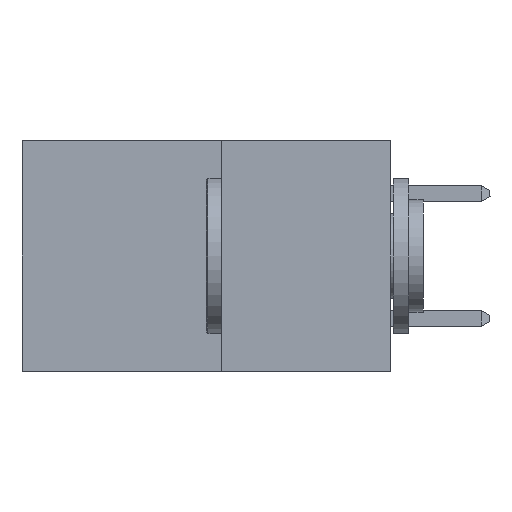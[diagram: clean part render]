
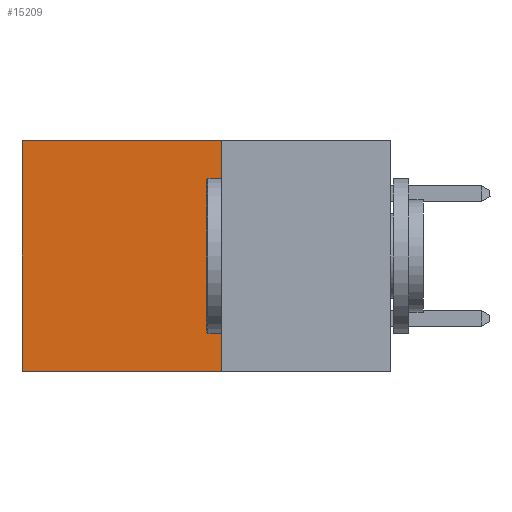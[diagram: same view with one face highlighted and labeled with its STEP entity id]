
A CAD part, left-side view. The second image highlights one B-rep face of the part: STEP entity #15209.
In plain terms, the highlighted planar face has unit normal (-1, 0, 0).
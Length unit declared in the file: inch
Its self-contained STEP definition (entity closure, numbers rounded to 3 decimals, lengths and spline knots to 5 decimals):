
#191 = DIRECTION ( 'NONE',  ( 0., 0., -1. ) ) ;
#684 = VERTEX_POINT ( 'NONE', #18938 ) ;
#930 = EDGE_CURVE ( 'NONE', #9327, #2776, #14267, .T. ) ;
#1476 = CARTESIAN_POINT ( 'NONE',  ( 0.277, 0.27, -0.37 ) ) ;
#1671 = AXIS2_PLACEMENT_3D ( 'NONE', #7876, #18685, #9533 ) ;
#2776 = VERTEX_POINT ( 'NONE', #19383 ) ;
#2973 = CARTESIAN_POINT ( 'NONE',  ( 0.277, 0.27, -0.37 ) ) ;
#4541 = CARTESIAN_POINT ( 'NONE',  ( 0.277, 0.59, -0.37 ) ) ;
#4821 = FACE_OUTER_BOUND ( 'NONE', #18161, .T. ) ;
#5572 = CARTESIAN_POINT ( 'NONE',  ( 0.277, 0.27, 0. ) ) ;
#5618 = VECTOR ( 'NONE', #17061, 39.37008 ) ;
#6107 = LINE ( 'NONE', #5572, #17521 ) ;
#6290 = EDGE_CURVE ( 'NONE', #8959, #9327, #7683, .T. ) ;
#7048 = ORIENTED_EDGE ( 'NONE', *, *, #13373, .T. ) ;
#7562 = ORIENTED_EDGE ( 'NONE', *, *, #930, .F. ) ;
#7656 = ORIENTED_EDGE ( 'NONE', *, *, #6290, .F. ) ;
#7683 = LINE ( 'NONE', #2973, #15938 ) ;
#7876 = CARTESIAN_POINT ( 'NONE',  ( 0.277, 0.27, -0.37 ) ) ;
#8193 = ORIENTED_EDGE ( 'NONE', *, *, #14936, .T. ) ;
#8959 = VERTEX_POINT ( 'NONE', #10296 ) ;
#9327 = VERTEX_POINT ( 'NONE', #1476 ) ;
#9533 = DIRECTION ( 'NONE',  ( 0., 0., -1. ) ) ;
#10296 = CARTESIAN_POINT ( 'NONE',  ( 0.277, 0.27, 0. ) ) ;
#11972 = DIRECTION ( 'NONE',  ( 0., 1., 0. ) ) ;
#13373 = EDGE_CURVE ( 'NONE', #684, #2776, #18020, .T. ) ;
#14054 = PLANE ( 'NONE',  #1671 ) ;
#14267 = LINE ( 'NONE', #19046, #14760 ) ;
#14760 = VECTOR ( 'NONE', #14883, 39.37008 ) ;
#14883 = DIRECTION ( 'NONE',  ( 0., 1., 0. ) ) ;
#14936 = EDGE_CURVE ( 'NONE', #8959, #684, #6107, .T. ) ;
#15209 = ADVANCED_FACE ( 'NONE', ( #4821 ), #14054, .F. ) ;
#15938 = VECTOR ( 'NONE', #191, 39.37008 ) ;
#17061 = DIRECTION ( 'NONE',  ( 0., 0., -1. ) ) ;
#17521 = VECTOR ( 'NONE', #11972, 39.37008 ) ;
#18020 = LINE ( 'NONE', #4541, #5618 ) ;
#18161 = EDGE_LOOP ( 'NONE', ( #7048, #7562, #7656, #8193 ) ) ;
#18685 = DIRECTION ( 'NONE',  ( 1., 0., 0. ) ) ;
#18938 = CARTESIAN_POINT ( 'NONE',  ( 0.277, 0.59, 0. ) ) ;
#19046 = CARTESIAN_POINT ( 'NONE',  ( 0.277, 0.27, -0.37 ) ) ;
#19383 = CARTESIAN_POINT ( 'NONE',  ( 0.277, 0.59, -0.37 ) ) ;
